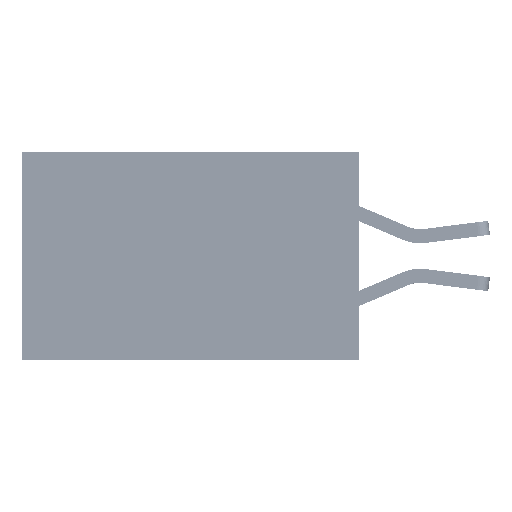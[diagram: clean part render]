
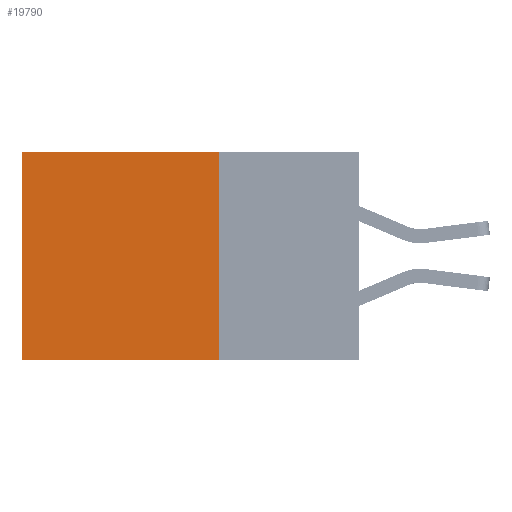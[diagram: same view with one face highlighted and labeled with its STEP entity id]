
A CAD part, left-side view. The second image highlights one B-rep face of the part: STEP entity #19790.
In plain terms, the highlighted planar face has unit normal (-1, 0, 0).
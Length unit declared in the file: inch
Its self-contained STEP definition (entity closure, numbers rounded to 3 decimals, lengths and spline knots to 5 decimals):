
#827 = EDGE_CURVE ( 'NONE', #16265, #18958, #14718, .T. ) ;
#1169 = AXIS2_PLACEMENT_3D ( 'NONE', #20244, #28961, #5517 ) ;
#3053 = EDGE_CURVE ( 'NONE', #20499, #16265, #37205, .T. ) ;
#4153 = EDGE_LOOP ( 'NONE', ( #37861, #13642, #32563, #35851 ) ) ;
#5517 = DIRECTION ( 'NONE',  ( 0., 0., -1. ) ) ;
#6192 = CARTESIAN_POINT ( 'NONE',  ( 0.2875, 0.25, -0.37 ) ) ;
#6225 = VECTOR ( 'NONE', #37155, 39.37008 ) ;
#7177 = VECTOR ( 'NONE', #15119, 39.37008 ) ;
#8742 = EDGE_CURVE ( 'NONE', #20499, #10721, #34436, .T. ) ;
#9548 = CARTESIAN_POINT ( 'NONE',  ( 0.2875, 0.25, -0.37 ) ) ;
#10651 = CARTESIAN_POINT ( 'NONE',  ( 0.2875, 0.25, 0. ) ) ;
#10721 = VERTEX_POINT ( 'NONE', #9548 ) ;
#11130 = LINE ( 'NONE', #6192, #7177 ) ;
#11269 = CARTESIAN_POINT ( 'NONE',  ( 0.2875, 0.6, -0.37 ) ) ;
#11700 = PLANE ( 'NONE',  #1169 ) ;
#13642 = ORIENTED_EDGE ( 'NONE', *, *, #17050, .F. ) ;
#14641 = CARTESIAN_POINT ( 'NONE',  ( 0.2875, 0.6, 0. ) ) ;
#14718 = LINE ( 'NONE', #32722, #18109 ) ;
#15119 = DIRECTION ( 'NONE',  ( 0., 1., 0. ) ) ;
#16096 = CARTESIAN_POINT ( 'NONE',  ( 0.2875, 0.25, 0. ) ) ;
#16265 = VERTEX_POINT ( 'NONE', #14641 ) ;
#17050 = EDGE_CURVE ( 'NONE', #10721, #18958, #11130, .T. ) ;
#18109 = VECTOR ( 'NONE', #26540, 39.37008 ) ;
#18958 = VERTEX_POINT ( 'NONE', #11269 ) ;
#19023 = VECTOR ( 'NONE', #34289, 39.37008 ) ;
#19790 = ADVANCED_FACE ( 'NONE', ( #35149 ), #11700, .F. ) ;
#20244 = CARTESIAN_POINT ( 'NONE',  ( 0.2875, 0.25, 0. ) ) ;
#20499 = VERTEX_POINT ( 'NONE', #16096 ) ;
#26540 = DIRECTION ( 'NONE',  ( 0., 0., -1. ) ) ;
#28961 = DIRECTION ( 'NONE',  ( 1., 0., 0. ) ) ;
#32563 = ORIENTED_EDGE ( 'NONE', *, *, #8742, .F. ) ;
#32722 = CARTESIAN_POINT ( 'NONE',  ( 0.2875, 0.6, 0. ) ) ;
#34289 = DIRECTION ( 'NONE',  ( 0., 1., 0. ) ) ;
#34436 = LINE ( 'NONE', #36758, #6225 ) ;
#35149 = FACE_OUTER_BOUND ( 'NONE', #4153, .T. ) ;
#35851 = ORIENTED_EDGE ( 'NONE', *, *, #3053, .T. ) ;
#36758 = CARTESIAN_POINT ( 'NONE',  ( 0.2875, 0.25, 0. ) ) ;
#37155 = DIRECTION ( 'NONE',  ( 0., 0., -1. ) ) ;
#37205 = LINE ( 'NONE', #10651, #19023 ) ;
#37861 = ORIENTED_EDGE ( 'NONE', *, *, #827, .T. ) ;
